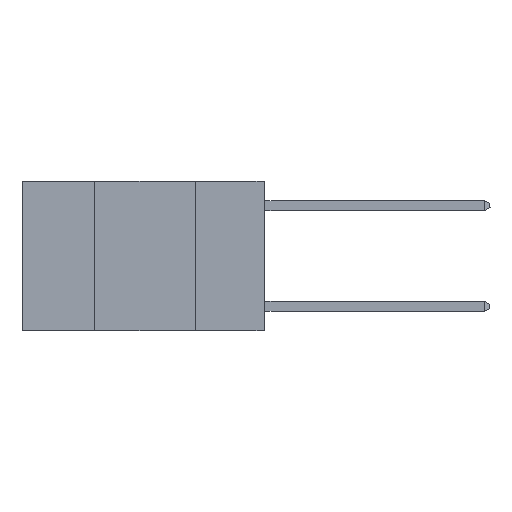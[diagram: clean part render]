
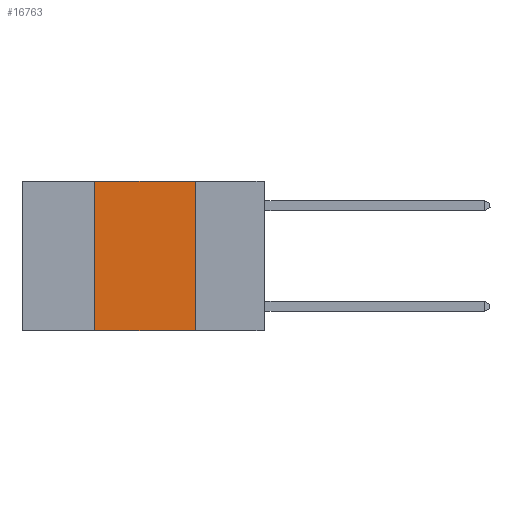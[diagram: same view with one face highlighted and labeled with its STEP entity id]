
A CAD part, left-side view. The second image highlights one B-rep face of the part: STEP entity #16763.
In plain terms, the highlighted planar face has unit normal (-1, 0, 0).
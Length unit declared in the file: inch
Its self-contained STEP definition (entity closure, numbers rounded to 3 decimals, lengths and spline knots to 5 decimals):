
#926 = VECTOR ( 'NONE', #15559, 39.37008 ) ;
#1150 = ORIENTED_EDGE ( 'NONE', *, *, #4341, .T. ) ;
#1418 = PLANE ( 'NONE',  #17203 ) ;
#2372 = CARTESIAN_POINT ( 'NONE',  ( 0., 0.17, 0. ) ) ;
#2906 = ORIENTED_EDGE ( 'NONE', *, *, #15712, .F. ) ;
#3679 = DIRECTION ( 'NONE',  ( 1., 0., 0. ) ) ;
#4341 = EDGE_CURVE ( 'NONE', #23602, #21385, #18747, .T. ) ;
#4474 = CARTESIAN_POINT ( 'NONE',  ( 0., 0.42, 0. ) ) ;
#4651 = DIRECTION ( 'NONE',  ( 0., 0., -1. ) ) ;
#4806 = CARTESIAN_POINT ( 'NONE',  ( 0., 0.17, 0. ) ) ;
#5226 = EDGE_LOOP ( 'NONE', ( #9165, #7436, #2906, #1150 ) ) ;
#5478 = VECTOR ( 'NONE', #4651, 39.37008 ) ;
#5676 = EDGE_CURVE ( 'NONE', #24177, #21385, #11376, .T. ) ;
#6879 = VERTEX_POINT ( 'NONE', #21991 ) ;
#7436 = ORIENTED_EDGE ( 'NONE', *, *, #21180, .F. ) ;
#7571 = LINE ( 'NONE', #4474, #926 ) ;
#8549 = FACE_OUTER_BOUND ( 'NONE', #5226, .T. ) ;
#8671 = CARTESIAN_POINT ( 'NONE',  ( 0., 0.6, -0.37 ) ) ;
#9165 = ORIENTED_EDGE ( 'NONE', *, *, #5676, .F. ) ;
#10123 = CARTESIAN_POINT ( 'NONE',  ( 0., 0.6, 0. ) ) ;
#10526 = LINE ( 'NONE', #10123, #11223 ) ;
#10905 = CARTESIAN_POINT ( 'NONE',  ( 0., 0.17, -0.37 ) ) ;
#11223 = VECTOR ( 'NONE', #27728, 39.37008 ) ;
#11376 = LINE ( 'NONE', #2372, #5478 ) ;
#12801 = VECTOR ( 'NONE', #28516, 39.37008 ) ;
#15559 = DIRECTION ( 'NONE',  ( 0., 0., 1. ) ) ;
#15712 = EDGE_CURVE ( 'NONE', #23602, #6879, #7571, .T. ) ;
#16513 = CARTESIAN_POINT ( 'NONE',  ( 0., 0.42, -0.37 ) ) ;
#16763 = ADVANCED_FACE ( 'NONE', ( #8549 ), #1418, .F. ) ;
#17028 = CARTESIAN_POINT ( 'NONE',  ( 0., 0.6, 0. ) ) ;
#17203 = AXIS2_PLACEMENT_3D ( 'NONE', #17028, #3679, #19282 ) ;
#18747 = LINE ( 'NONE', #8671, #12801 ) ;
#19282 = DIRECTION ( 'NONE',  ( 0., 0., -1. ) ) ;
#21180 = EDGE_CURVE ( 'NONE', #6879, #24177, #10526, .T. ) ;
#21385 = VERTEX_POINT ( 'NONE', #10905 ) ;
#21991 = CARTESIAN_POINT ( 'NONE',  ( 0., 0.42, 0. ) ) ;
#23602 = VERTEX_POINT ( 'NONE', #16513 ) ;
#24177 = VERTEX_POINT ( 'NONE', #4806 ) ;
#27728 = DIRECTION ( 'NONE',  ( 0., -1., 0. ) ) ;
#28516 = DIRECTION ( 'NONE',  ( 0., -1., 0. ) ) ;
